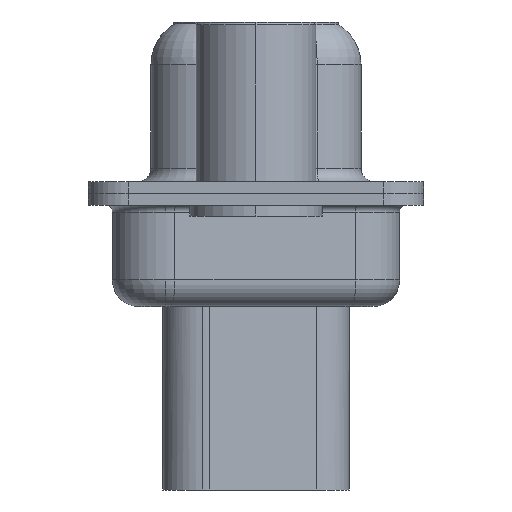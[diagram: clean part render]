
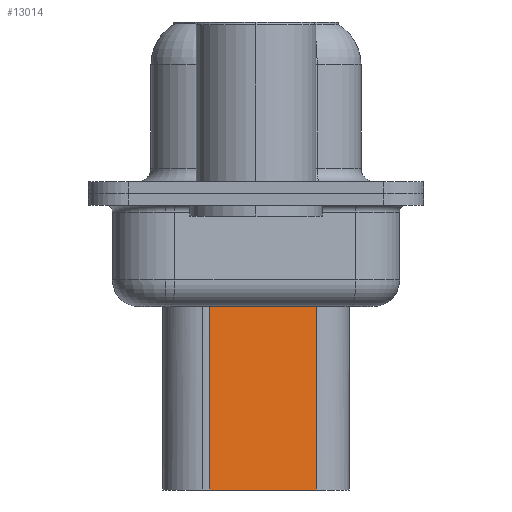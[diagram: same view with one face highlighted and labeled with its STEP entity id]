
A CAD part, left-side view. The second image highlights one B-rep face of the part: STEP entity #13014.
In plain terms, the highlighted planar face has unit normal (-0.985, -0.174, 0).
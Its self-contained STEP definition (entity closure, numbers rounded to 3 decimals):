
#1654 = EDGE_CURVE ( 'NONE', #12802, #7914, #12299, .T. ) ;
#1812 = DIRECTION ( 'NONE',  ( 0., 0., -1. ) ) ;
#3011 = CARTESIAN_POINT ( 'NONE',  ( 5.229, -2.26, -11.15 ) ) ;
#3018 = DIRECTION ( 'NONE',  ( -0.174, 0.985, 0. ) ) ;
#3277 = EDGE_CURVE ( 'NONE', #6952, #10801, #6312, .T. ) ;
#3914 = VECTOR ( 'NONE', #1812, 1000. ) ;
#4141 = DIRECTION ( 'NONE',  ( -0.174, 0.985, 0. ) ) ;
#5044 = VECTOR ( 'NONE', #8508, 1000. ) ;
#5231 = CARTESIAN_POINT ( 'NONE',  ( 5.229, -2.26, -3.975 ) ) ;
#5567 = ORIENTED_EDGE ( 'NONE', *, *, #1654, .F. ) ;
#5804 = ORIENTED_EDGE ( 'NONE', *, *, #3277, .T. ) ;
#6312 = LINE ( 'NONE', #11543, #7063 ) ;
#6925 = EDGE_CURVE ( 'NONE', #10801, #7914, #10013, .T. ) ;
#6952 = VERTEX_POINT ( 'NONE', #5231 ) ;
#7063 = VECTOR ( 'NONE', #4141, 1000. ) ;
#7204 = CARTESIAN_POINT ( 'NONE',  ( 4.524, 1.74, -11.15 ) ) ;
#7270 = CARTESIAN_POINT ( 'NONE',  ( 4.524, 1.74, -3.1 ) ) ;
#7398 = PLANE ( 'NONE',  #13138 ) ;
#7686 = CARTESIAN_POINT ( 'NONE',  ( 4.524, 1.74, -3.975 ) ) ;
#7914 = VERTEX_POINT ( 'NONE', #9081 ) ;
#8381 = LINE ( 'NONE', #9386, #5044 ) ;
#8419 = DIRECTION ( 'NONE',  ( 0.174, -0.985, 0. ) ) ;
#8422 = EDGE_CURVE ( 'NONE', #6952, #12802, #8381, .T. ) ;
#8508 = DIRECTION ( 'NONE',  ( 0., 0., -1. ) ) ;
#8560 = CARTESIAN_POINT ( 'NONE',  ( 4.524, 1.74, -3.1 ) ) ;
#8685 = FACE_OUTER_BOUND ( 'NONE', #11340, .T. ) ;
#8872 = ORIENTED_EDGE ( 'NONE', *, *, #6925, .T. ) ;
#9081 = CARTESIAN_POINT ( 'NONE',  ( 4.524, 1.74, -11.15 ) ) ;
#9386 = CARTESIAN_POINT ( 'NONE',  ( 5.229, -2.26, -3.1 ) ) ;
#9641 = DIRECTION ( 'NONE',  ( -0.985, -0.174, 0. ) ) ;
#10013 = LINE ( 'NONE', #7270, #3914 ) ;
#10801 = VERTEX_POINT ( 'NONE', #7686 ) ;
#11170 = ORIENTED_EDGE ( 'NONE', *, *, #8422, .F. ) ;
#11340 = EDGE_LOOP ( 'NONE', ( #11170, #5804, #8872, #5567 ) ) ;
#11543 = CARTESIAN_POINT ( 'NONE',  ( 4.353, 2.709, -3.975 ) ) ;
#12116 = VECTOR ( 'NONE', #3018, 1000. ) ;
#12299 = LINE ( 'NONE', #7204, #12116 ) ;
#12802 = VERTEX_POINT ( 'NONE', #3011 ) ;
#13014 = ADVANCED_FACE ( 'NONE', ( #8685 ), #7398, .T. ) ;
#13138 = AXIS2_PLACEMENT_3D ( 'NONE', #8560, #9641, #8419 ) ;
